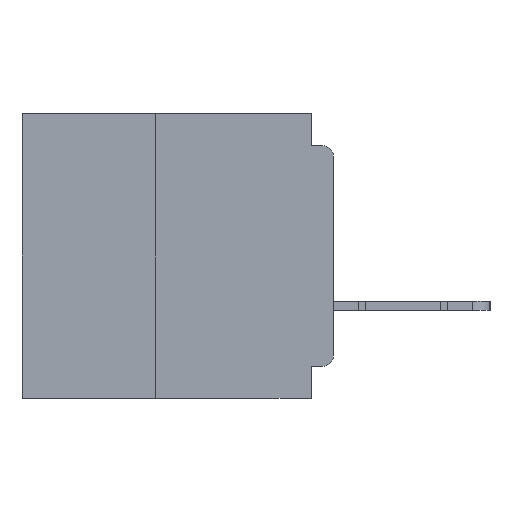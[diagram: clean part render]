
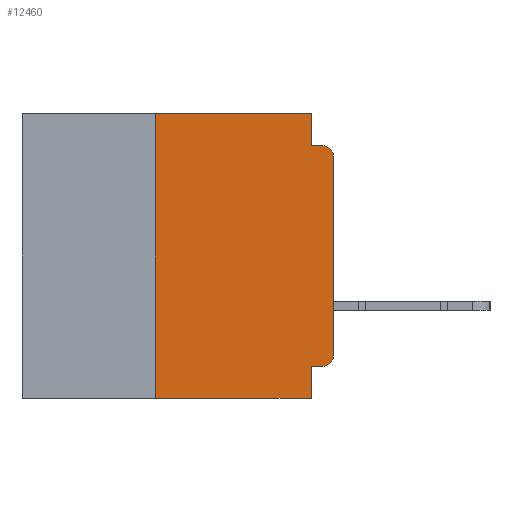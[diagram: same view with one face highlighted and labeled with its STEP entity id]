
A CAD part, left-side view. The second image highlights one B-rep face of the part: STEP entity #12460.
In plain terms, the highlighted planar face has unit normal (-1, 0, 0).
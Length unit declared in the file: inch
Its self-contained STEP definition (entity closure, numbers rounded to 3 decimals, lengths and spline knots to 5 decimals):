
#555 = CARTESIAN_POINT ( 'NONE',  ( 0., 0., -0.045 ) ) ;
#1942 = CARTESIAN_POINT ( 'NONE',  ( 0., 0.031, -0.4 ) ) ;
#3361 = CARTESIAN_POINT ( 'NONE',  ( 0., 0.25, 0. ) ) ;
#3526 = VECTOR ( 'NONE', #62304, 39.37008 ) ;
#3795 = LINE ( 'NONE', #555, #26797 ) ;
#4692 = DIRECTION ( 'NONE',  ( 0., -1., 0. ) ) ;
#5330 = ORIENTED_EDGE ( 'NONE', *, *, #15416, .F. ) ;
#6307 = LINE ( 'NONE', #36691, #32471 ) ;
#6405 = ORIENTED_EDGE ( 'NONE', *, *, #27409, .F. ) ;
#6682 = CARTESIAN_POINT ( 'NONE',  ( 0., 0., -0.355 ) ) ;
#7188 = VERTEX_POINT ( 'NONE', #44645 ) ;
#7237 = DIRECTION ( 'NONE',  ( 0., 0., -1. ) ) ;
#8103 = PLANE ( 'NONE',  #40257 ) ;
#10897 = VERTEX_POINT ( 'NONE', #26008 ) ;
#11903 = ORIENTED_EDGE ( 'NONE', *, *, #16238, .F. ) ;
#12375 = CARTESIAN_POINT ( 'NONE',  ( 0., 0.031, -0.045 ) ) ;
#12460 = ADVANCED_FACE ( 'NONE', ( #55540 ), #8103, .F. ) ;
#14795 = VERTEX_POINT ( 'NONE', #12375 ) ;
#14881 = EDGE_CURVE ( 'NONE', #24762, #54892, #53474, .T. ) ;
#15416 = EDGE_CURVE ( 'NONE', #25755, #29559, #22728, .T. ) ;
#16238 = EDGE_CURVE ( 'NONE', #14795, #54892, #3795, .T. ) ;
#16266 = CARTESIAN_POINT ( 'NONE',  ( 0., 0.015, -0.355 ) ) ;
#16508 = CARTESIAN_POINT ( 'NONE',  ( 0., 0.437, 0. ) ) ;
#16930 = CARTESIAN_POINT ( 'NONE',  ( 0., 0.015, -0.045 ) ) ;
#17967 = EDGE_CURVE ( 'NONE', #64735, #24762, #45076, .T. ) ;
#18604 = CARTESIAN_POINT ( 'NONE',  ( 0., 0.015, -0.06 ) ) ;
#18616 = EDGE_CURVE ( 'NONE', #24013, #64735, #28880, .T. ) ;
#20468 = EDGE_CURVE ( 'NONE', #24013, #25755, #49581, .T. ) ;
#21058 = VECTOR ( 'NONE', #7237, 39.37008 ) ;
#21305 = LINE ( 'NONE', #16508, #60890 ) ;
#22214 = EDGE_LOOP ( 'NONE', ( #40370, #30701, #11903, #23530, #37519, #6405, #48769, #5330, #36792, #54876 ) ) ;
#22728 = LINE ( 'NONE', #1942, #21058 ) ;
#23530 = ORIENTED_EDGE ( 'NONE', *, *, #23974, .F. ) ;
#23877 = DIRECTION ( 'NONE',  ( 0., 0., -1. ) ) ;
#23974 = EDGE_CURVE ( 'NONE', #10897, #14795, #6307, .T. ) ;
#23984 = DIRECTION ( 'NONE',  ( 0., 0., -1. ) ) ;
#24013 = VERTEX_POINT ( 'NONE', #16266 ) ;
#24762 = VERTEX_POINT ( 'NONE', #53279 ) ;
#25364 = CARTESIAN_POINT ( 'NONE',  ( 0., 0.25, -0.4 ) ) ;
#25755 = VERTEX_POINT ( 'NONE', #30858 ) ;
#26008 = CARTESIAN_POINT ( 'NONE',  ( 0., 0.031, 0. ) ) ;
#26232 = DIRECTION ( 'NONE',  ( -1., 0., 0. ) ) ;
#26797 = VECTOR ( 'NONE', #62725, 39.37008 ) ;
#27409 = EDGE_CURVE ( 'NONE', #7188, #33038, #50541, .T. ) ;
#28289 = EDGE_CURVE ( 'NONE', #33038, #10897, #21305, .T. ) ;
#28497 = CARTESIAN_POINT ( 'NONE',  ( 0., 0.031, -0.4 ) ) ;
#28880 = CIRCLE ( 'NONE', #41853, 0.015 ) ;
#29559 = VERTEX_POINT ( 'NONE', #28497 ) ;
#30701 = ORIENTED_EDGE ( 'NONE', *, *, #14881, .T. ) ;
#30858 = CARTESIAN_POINT ( 'NONE',  ( 0., 0.031, -0.355 ) ) ;
#32471 = VECTOR ( 'NONE', #52265, 39.37008 ) ;
#32534 = VECTOR ( 'NONE', #4692, 39.37008 ) ;
#33038 = VERTEX_POINT ( 'NONE', #3361 ) ;
#34210 = VECTOR ( 'NONE', #37873, 39.37008 ) ;
#35931 = CARTESIAN_POINT ( 'NONE',  ( 0., 0.437, -0.4 ) ) ;
#36691 = CARTESIAN_POINT ( 'NONE',  ( 0., 0.031, 0. ) ) ;
#36792 = ORIENTED_EDGE ( 'NONE', *, *, #20468, .F. ) ;
#37519 = ORIENTED_EDGE ( 'NONE', *, *, #28289, .F. ) ;
#37873 = DIRECTION ( 'NONE',  ( 0., 1., 0. ) ) ;
#40257 = AXIS2_PLACEMENT_3D ( 'NONE', #49707, #54860, #23984 ) ;
#40370 = ORIENTED_EDGE ( 'NONE', *, *, #17967, .T. ) ;
#41853 = AXIS2_PLACEMENT_3D ( 'NONE', #57099, #26232, #62216 ) ;
#44645 = CARTESIAN_POINT ( 'NONE',  ( 0., 0.25, -0.4 ) ) ;
#44978 = EDGE_CURVE ( 'NONE', #7188, #29559, #46264, .T. ) ;
#45076 = LINE ( 'NONE', #57178, #3526 ) ;
#46264 = LINE ( 'NONE', #35931, #32534 ) ;
#47778 = DIRECTION ( 'NONE',  ( 0., -1., 0. ) ) ;
#48769 = ORIENTED_EDGE ( 'NONE', *, *, #44978, .T. ) ;
#49581 = LINE ( 'NONE', #6682, #34210 ) ;
#49707 = CARTESIAN_POINT ( 'NONE',  ( 0., 0.437, 0. ) ) ;
#50541 = LINE ( 'NONE', #25364, #65817 ) ;
#51251 = CARTESIAN_POINT ( 'NONE',  ( 0., 0., -0.34 ) ) ;
#52265 = DIRECTION ( 'NONE',  ( 0., 0., -1. ) ) ;
#53279 = CARTESIAN_POINT ( 'NONE',  ( 0., 0., -0.06 ) ) ;
#53474 = CIRCLE ( 'NONE', #61985, 0.015 ) ;
#54757 = DIRECTION ( 'NONE',  ( -1., 0., 0. ) ) ;
#54860 = DIRECTION ( 'NONE',  ( 1., 0., 0. ) ) ;
#54876 = ORIENTED_EDGE ( 'NONE', *, *, #18616, .T. ) ;
#54892 = VERTEX_POINT ( 'NONE', #16930 ) ;
#55540 = FACE_OUTER_BOUND ( 'NONE', #22214, .T. ) ;
#57099 = CARTESIAN_POINT ( 'NONE',  ( 0., 0.015, -0.34 ) ) ;
#57178 = CARTESIAN_POINT ( 'NONE',  ( 0., 0., 0. ) ) ;
#60890 = VECTOR ( 'NONE', #47778, 39.37008 ) ;
#61378 = DIRECTION ( 'NONE',  ( 0., 0., 1. ) ) ;
#61985 = AXIS2_PLACEMENT_3D ( 'NONE', #18604, #54757, #23877 ) ;
#62216 = DIRECTION ( 'NONE',  ( 0., 0., -1. ) ) ;
#62304 = DIRECTION ( 'NONE',  ( 0., 0., 1. ) ) ;
#62725 = DIRECTION ( 'NONE',  ( 0., -1., 0. ) ) ;
#64735 = VERTEX_POINT ( 'NONE', #51251 ) ;
#65817 = VECTOR ( 'NONE', #61378, 39.37008 ) ;
